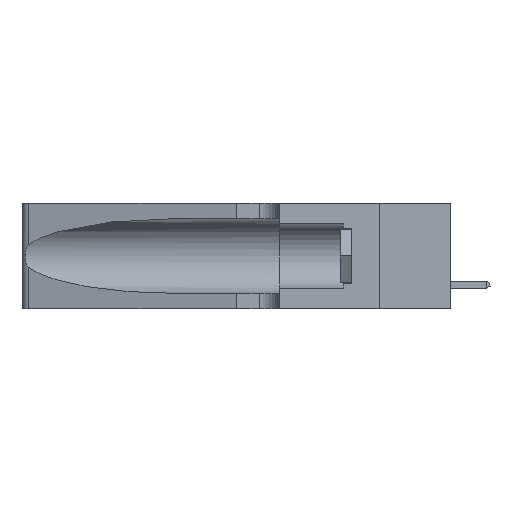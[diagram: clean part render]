
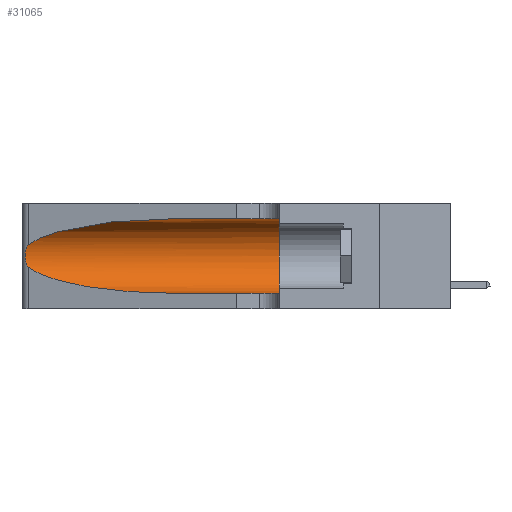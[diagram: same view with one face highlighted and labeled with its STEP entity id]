
A CAD part, left-side view. The second image highlights one B-rep face of the part: STEP entity #31065.
In plain terms, the highlighted cylindrical face has radius 3.308 mm (diameter 6.617 mm), a partial arc.
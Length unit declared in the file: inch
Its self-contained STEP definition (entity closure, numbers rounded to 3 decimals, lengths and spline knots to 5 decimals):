
#115 = ORIENTED_EDGE ( 'NONE', *, *, #29746, .T. ) ;
#612 = CARTESIAN_POINT ( 'NONE',  ( 0.1305, 0.72297, 0.05475 ) ) ;
#972 = CARTESIAN_POINT ( 'NONE',  ( 0.1305, 1.61858, 0.185 ) ) ;
#2437 = FACE_OUTER_BOUND ( 'NONE', #18006, .T. ) ;
#3664 = AXIS2_PLACEMENT_3D ( 'NONE', #972, #21481, #31575 ) ;
#3764 = CARTESIAN_POINT ( 'NONE',  ( 0.26017, 1.23833, 0.17102 ) ) ;
#3835 = ORIENTED_EDGE ( 'NONE', *, *, #37650, .T. ) ;
#4063 = CARTESIAN_POINT ( 'NONE',  ( 0.25787, 1.23484, 0.2124 ) ) ;
#4212 = CARTESIAN_POINT ( 'NONE',  ( 0.25487, 1.22718, 0.14631 ) ) ;
#4264 = CARTESIAN_POINT ( 'NONE',  ( 0.1305, 0.35, 0.05475 ) ) ;
#4538 = CYLINDRICAL_SURFACE ( 'NONE', #3664, 0.13025 ) ;
#4692 = ORIENTED_EDGE ( 'NONE', *, *, #21805, .F. ) ;
#5093 =( BOUNDED_CURVE ( )  B_SPLINE_CURVE ( 3, ( #7170, #34164, #14015, #612 ),
 .UNSPECIFIED., .F., .F. ) 
 B_SPLINE_CURVE_WITH_KNOTS ( ( 4, 4 ),
 ( 3.44316, 4.71239 ),
 .UNSPECIFIED. ) 
 CURVE ( )  GEOMETRIC_REPRESENTATION_ITEM ( )  RATIONAL_B_SPLINE_CURVE ( ( 1., 0.87, 0.87, 1. ) ) 
 REPRESENTATION_ITEM ( '' )  );
#5843 = CARTESIAN_POINT ( 'NONE',  ( 0.18966, 0.96281, 0.31525 ) ) ;
#6407 = CARTESIAN_POINT ( 'NONE',  ( 0.1305, 0.72297, 0.05475 ) ) ;
#7170 = CARTESIAN_POINT ( 'NONE',  ( 0.25487, 1.22718, 0.14631 ) ) ;
#7419 = CARTESIAN_POINT ( 'NONE',  ( 0.25487, 1.22718, 0.22369 ) ) ;
#7580 = CARTESIAN_POINT ( 'NONE',  ( 0.26075, 1.23896, 0.178 ) ) ;
#7799 = LINE ( 'NONE', #15733, #42678 ) ;
#8858 = VERTEX_POINT ( 'NONE', #6407 ) ;
#9503 = CARTESIAN_POINT ( 'NONE',  ( 0.2373, 1.15595, 0.28018 ) ) ;
#10185 = CARTESIAN_POINT ( 'NONE',  ( 0.25487, 1.22718, 0.14631 ) ) ;
#10258 = EDGE_CURVE ( 'NONE', #42966, #39229, #16138, .T. ) ;
#10793 = CARTESIAN_POINT ( 'NONE',  ( 0.25854, 1.2359, 0.20912 ) ) ;
#10937 = CARTESIAN_POINT ( 'NONE',  ( 0.25555, 1.22993, 0.14849 ) ) ;
#14015 = CARTESIAN_POINT ( 'NONE',  ( 0.18966, 0.96281, 0.05475 ) ) ;
#14139 = CARTESIAN_POINT ( 'NONE',  ( 0.26075, 1.23896, 0.19203 ) ) ;
#14385 = CARTESIAN_POINT ( 'NONE',  ( 0.1305, 0.72297, 0.31525 ) ) ;
#15733 = CARTESIAN_POINT ( 'NONE',  ( 0.1305, 1.61858, 0.31525 ) ) ;
#16138 =( BOUNDED_CURVE ( )  B_SPLINE_CURVE ( 3, ( #16391, #5843, #9503, #36482 ),
 .UNSPECIFIED., .F., .F. ) 
 B_SPLINE_CURVE_WITH_KNOTS ( ( 4, 4 ),
 ( 1.5708, 2.84003 ),
 .UNSPECIFIED. ) 
 CURVE ( )  GEOMETRIC_REPRESENTATION_ITEM ( )  RATIONAL_B_SPLINE_CURVE ( ( 1., 0.87, 0.87, 1. ) ) 
 REPRESENTATION_ITEM ( '' )  );
#16391 = CARTESIAN_POINT ( 'NONE',  ( 0.1305, 0.72297, 0.31525 ) ) ;
#17529 = CARTESIAN_POINT ( 'NONE',  ( 0.25789, 1.23486, 0.15765 ) ) ;
#18006 = EDGE_LOOP ( 'NONE', ( #27616, #35319, #115, #3835, #4692, #27464 ) ) ;
#18108 = LINE ( 'NONE', #27027, #36664 ) ;
#18809 = B_SPLINE_CURVE_WITH_KNOTS ( 'NONE', 3,
 ( #7419, #27225, #24389, #4063, #10793, #34434, #14139, #7580, #3764, #34023, #17529, #20973, #10937, #4212 ),
 .UNSPECIFIED., .F., .F.,
 ( 4, 2, 2, 2, 2, 2, 4 ),
 ( 0., 0.00027, 0.00053, 0.00107, 0.0016, 0.00187, 0.00214 ),
 .UNSPECIFIED. ) ;
#18829 = DIRECTION ( 'NONE',  ( 0., -1., 0. ) ) ;
#20973 = CARTESIAN_POINT ( 'NONE',  ( 0.25639, 1.23186, 0.15144 ) ) ;
#21481 = DIRECTION ( 'NONE',  ( 0., -1., 0. ) ) ;
#21805 = EDGE_CURVE ( 'NONE', #31045, #31056, #35231, .T. ) ;
#23415 = CARTESIAN_POINT ( 'NONE',  ( 0.25487, 1.22718, 0.22369 ) ) ;
#24389 = CARTESIAN_POINT ( 'NONE',  ( 0.25639, 1.23184, 0.21858 ) ) ;
#27027 = CARTESIAN_POINT ( 'NONE',  ( 0.1305, 1.61858, 0.05475 ) ) ;
#27225 = CARTESIAN_POINT ( 'NONE',  ( 0.25555, 1.22994, 0.2215 ) ) ;
#27464 = ORIENTED_EDGE ( 'NONE', *, *, #36067, .F. ) ;
#27616 = ORIENTED_EDGE ( 'NONE', *, *, #10258, .T. ) ;
#27998 = CARTESIAN_POINT ( 'NONE',  ( 0.1305, 0.35, 0.31525 ) ) ;
#29746 = EDGE_CURVE ( 'NONE', #40469, #8858, #5093, .T. ) ;
#30296 = DIRECTION ( 'NONE',  ( 0., -1., 0. ) ) ;
#31045 = VERTEX_POINT ( 'NONE', #27998 ) ;
#31056 = VERTEX_POINT ( 'NONE', #4264 ) ;
#31065 = ADVANCED_FACE ( 'NONE', ( #2437 ), #4538, .F. ) ;
#31575 = DIRECTION ( 'NONE',  ( 0., 0., -1. ) ) ;
#32199 = DIRECTION ( 'NONE',  ( 0., 0., 1. ) ) ;
#34023 = CARTESIAN_POINT ( 'NONE',  ( 0.25856, 1.23593, 0.16098 ) ) ;
#34164 = CARTESIAN_POINT ( 'NONE',  ( 0.2373, 1.15595, 0.08982 ) ) ;
#34434 = CARTESIAN_POINT ( 'NONE',  ( 0.26018, 1.23835, 0.19895 ) ) ;
#35231 = CIRCLE ( 'NONE', #36831, 0.13025 ) ;
#35319 = ORIENTED_EDGE ( 'NONE', *, *, #41083, .T. ) ;
#36067 = EDGE_CURVE ( 'NONE', #42966, #31045, #7799, .T. ) ;
#36144 = DIRECTION ( 'NONE',  ( 0., 1., 0. ) ) ;
#36482 = CARTESIAN_POINT ( 'NONE',  ( 0.25487, 1.22718, 0.22369 ) ) ;
#36664 = VECTOR ( 'NONE', #30296, 39.37008 ) ;
#36831 = AXIS2_PLACEMENT_3D ( 'NONE', #42772, #36144, #32199 ) ;
#37650 = EDGE_CURVE ( 'NONE', #8858, #31056, #18108, .T. ) ;
#39229 = VERTEX_POINT ( 'NONE', #23415 ) ;
#40469 = VERTEX_POINT ( 'NONE', #10185 ) ;
#41083 = EDGE_CURVE ( 'NONE', #39229, #40469, #18809, .T. ) ;
#42678 = VECTOR ( 'NONE', #18829, 39.37008 ) ;
#42772 = CARTESIAN_POINT ( 'NONE',  ( 0.1305, 0.35, 0.185 ) ) ;
#42966 = VERTEX_POINT ( 'NONE', #14385 ) ;
